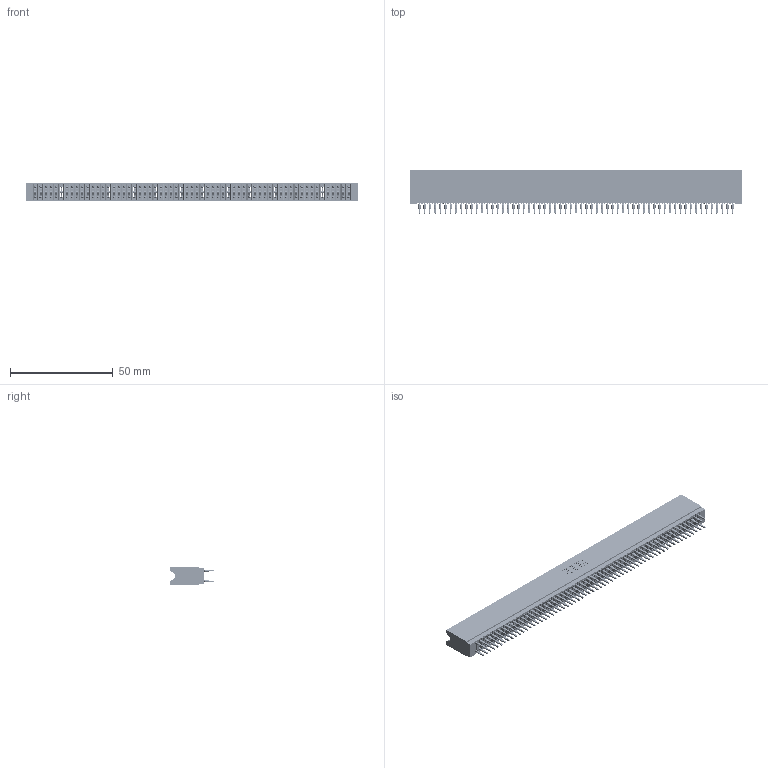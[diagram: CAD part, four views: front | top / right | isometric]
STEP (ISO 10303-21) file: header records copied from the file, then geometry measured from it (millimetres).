
FILE_DESCRIPTION (( 'STEP AP203' ), '1' );
FILE_NAME ('745-122-560-206.STEP', '2020-09-14T17:42:54', ( '' ), ( '' ), 'SwSTEP 2.0', 'SolidWorks 2020', '' );
FILE_SCHEMA (( 'CONFIG_CONTROL_DESIGN' ));
Products named in the file (3): 745-292-001_560; 745-122-560-206; 745 Part_Insulator Option - 06
Assembly tree (123 placements, depth 2):
  745-122-560-206
    745 Part_Insulator Option - 06
    745-292-001_560  x122
Bounding box: 161.54 x 21.22 x 8.89 mm (x, y, z)
Volume: 14862.1 mm3; surface area: 32605.1 mm2
Topology: 123 solids, 123 shells, 12113 faces, 33139 edges, 21034 vertices
Faces by surface type: plane 6278, cylinder 2663, bspline 2440, torus 732
Entity records: 100450 total; most frequent: CARTESIAN_POINT 17920, ORIENTED_EDGE 17394, DIRECTION 15183, EDGE_CURVE 8697, LINE 8141, VECTOR 8141, VERTEX_POINT 5546, AXIS2_PLACEMENT_3D 3521
